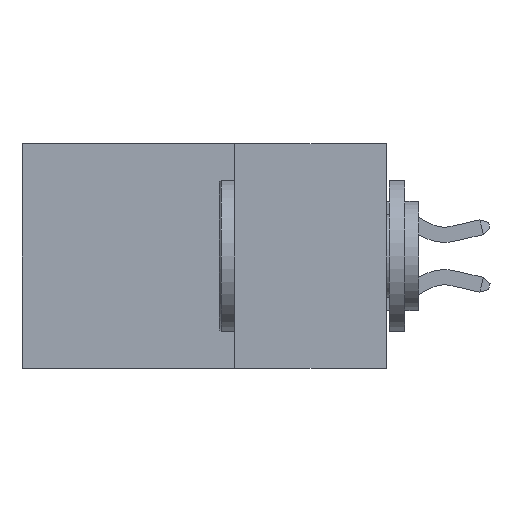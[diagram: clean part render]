
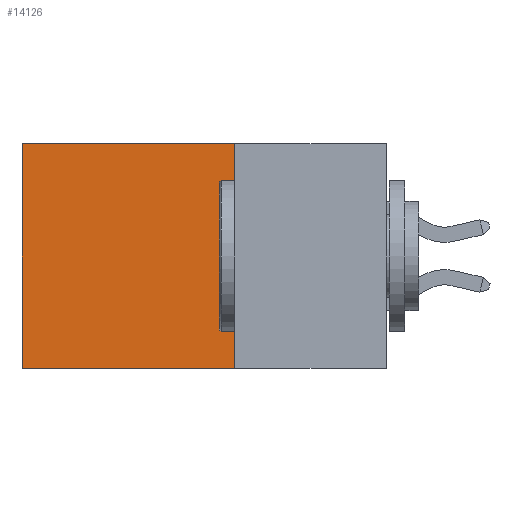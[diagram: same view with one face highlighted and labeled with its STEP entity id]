
A CAD part, left-side view. The second image highlights one B-rep face of the part: STEP entity #14126.
In plain terms, the highlighted planar face has unit normal (-1, 0, 0).
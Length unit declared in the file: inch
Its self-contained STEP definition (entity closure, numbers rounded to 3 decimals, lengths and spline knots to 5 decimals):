
#1142 = DIRECTION ( 'NONE',  ( 1., 0., 0. ) ) ;
#1353 = EDGE_CURVE ( 'NONE', #9367, #18654, #3093, .T. ) ;
#2602 = VECTOR ( 'NONE', #3016, 39.37008 ) ;
#2775 = PLANE ( 'NONE',  #20739 ) ;
#3016 = DIRECTION ( 'NONE',  ( 0., 1., 0. ) ) ;
#3093 = LINE ( 'NONE', #4328, #11545 ) ;
#4328 = CARTESIAN_POINT ( 'NONE',  ( 0.2615, 0.25, -0.37 ) ) ;
#5030 = DIRECTION ( 'NONE',  ( 0., 0., -1. ) ) ;
#5971 = VERTEX_POINT ( 'NONE', #6335 ) ;
#6175 = VECTOR ( 'NONE', #5030, 39.37008 ) ;
#6252 = CARTESIAN_POINT ( 'NONE',  ( 0.2615, 0.25, -0.37 ) ) ;
#6335 = CARTESIAN_POINT ( 'NONE',  ( 0.2615, 0.6, 0. ) ) ;
#7726 = EDGE_CURVE ( 'NONE', #5971, #11440, #14986, .T. ) ;
#7975 = DIRECTION ( 'NONE',  ( 0., 1., 0. ) ) ;
#8766 = ORIENTED_EDGE ( 'NONE', *, *, #7726, .T. ) ;
#9299 = FACE_OUTER_BOUND ( 'NONE', #10344, .T. ) ;
#9367 = VERTEX_POINT ( 'NONE', #12342 ) ;
#9873 = LINE ( 'NONE', #6252, #17900 ) ;
#10344 = EDGE_LOOP ( 'NONE', ( #8766, #14472, #16124, #18179 ) ) ;
#11269 = CARTESIAN_POINT ( 'NONE',  ( 0.2615, 0.25, -0.37 ) ) ;
#11440 = VERTEX_POINT ( 'NONE', #13935 ) ;
#11545 = VECTOR ( 'NONE', #18955, 39.37008 ) ;
#12342 = CARTESIAN_POINT ( 'NONE',  ( 0.2615, 0.25, 0. ) ) ;
#12934 = DIRECTION ( 'NONE',  ( 0., 0., -1. ) ) ;
#13397 = CARTESIAN_POINT ( 'NONE',  ( 0.2615, 0.6, -0.37 ) ) ;
#13589 = CARTESIAN_POINT ( 'NONE',  ( 0.2615, 0.25, -0.37 ) ) ;
#13935 = CARTESIAN_POINT ( 'NONE',  ( 0.2615, 0.6, -0.37 ) ) ;
#14126 = ADVANCED_FACE ( 'NONE', ( #9299 ), #2775, .F. ) ;
#14472 = ORIENTED_EDGE ( 'NONE', *, *, #20889, .F. ) ;
#14700 = CARTESIAN_POINT ( 'NONE',  ( 0.2615, 0.25, 0. ) ) ;
#14986 = LINE ( 'NONE', #13397, #6175 ) ;
#15504 = EDGE_CURVE ( 'NONE', #9367, #5971, #15834, .T. ) ;
#15834 = LINE ( 'NONE', #14700, #2602 ) ;
#16124 = ORIENTED_EDGE ( 'NONE', *, *, #1353, .F. ) ;
#17900 = VECTOR ( 'NONE', #7975, 39.37008 ) ;
#18179 = ORIENTED_EDGE ( 'NONE', *, *, #15504, .T. ) ;
#18654 = VERTEX_POINT ( 'NONE', #13589 ) ;
#18955 = DIRECTION ( 'NONE',  ( 0., 0., -1. ) ) ;
#20739 = AXIS2_PLACEMENT_3D ( 'NONE', #11269, #1142, #12934 ) ;
#20889 = EDGE_CURVE ( 'NONE', #18654, #11440, #9873, .T. ) ;
